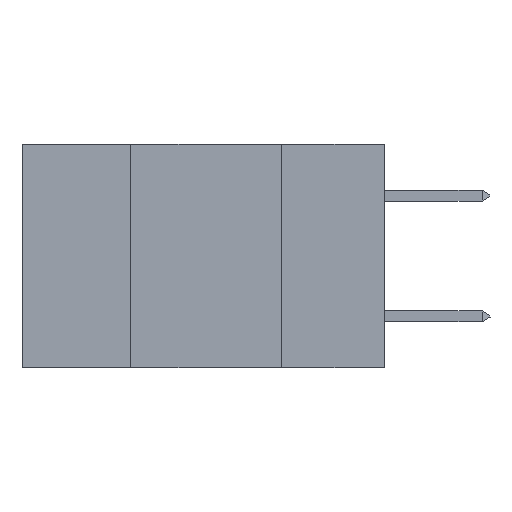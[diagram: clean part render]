
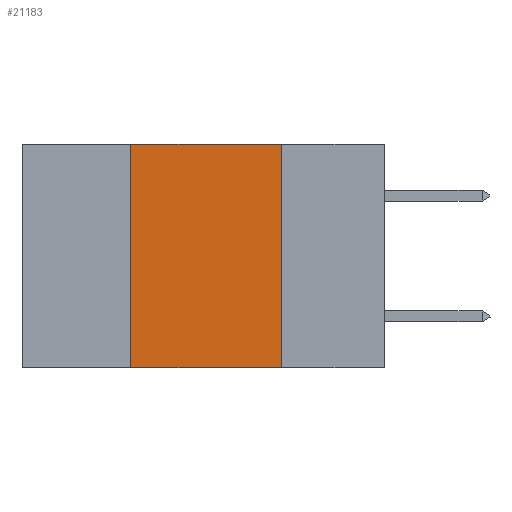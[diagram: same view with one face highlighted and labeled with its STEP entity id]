
A CAD part, left-side view. The second image highlights one B-rep face of the part: STEP entity #21183.
In plain terms, the highlighted planar face has unit normal (-1, 0, 0).
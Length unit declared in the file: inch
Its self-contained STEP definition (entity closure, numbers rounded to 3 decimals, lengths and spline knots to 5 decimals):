
#205 = DIRECTION ( 'NONE',  ( 0., 0., 1. ) ) ;
#1517 = VERTEX_POINT ( 'NONE', #17051 ) ;
#1685 = LINE ( 'NONE', #21232, #7131 ) ;
#1916 = CARTESIAN_POINT ( 'NONE',  ( 0., 0.6, 0. ) ) ;
#2679 = CARTESIAN_POINT ( 'NONE',  ( 0., 0.17, 0. ) ) ;
#4325 = CARTESIAN_POINT ( 'NONE',  ( 0., 0.6, -0.37 ) ) ;
#4379 = ORIENTED_EDGE ( 'NONE', *, *, #7152, .F. ) ;
#6887 = ORIENTED_EDGE ( 'NONE', *, *, #26153, .T. ) ;
#7084 = FACE_OUTER_BOUND ( 'NONE', #20321, .T. ) ;
#7131 = VECTOR ( 'NONE', #15181, 39.37008 ) ;
#7152 = EDGE_CURVE ( 'NONE', #16891, #16046, #12482, .T. ) ;
#7318 = CARTESIAN_POINT ( 'NONE',  ( 0., 0.42, -0.37 ) ) ;
#9005 = LINE ( 'NONE', #14502, #18321 ) ;
#10237 = VERTEX_POINT ( 'NONE', #7318 ) ;
#11109 = EDGE_CURVE ( 'NONE', #16046, #1517, #1685, .T. ) ;
#12009 = EDGE_CURVE ( 'NONE', #10237, #16891, #9005, .T. ) ;
#12128 = DIRECTION ( 'NONE',  ( 1., 0., 0. ) ) ;
#12482 = LINE ( 'NONE', #1916, #14392 ) ;
#13157 = AXIS2_PLACEMENT_3D ( 'NONE', #20233, #12128, #15914 ) ;
#13162 = CARTESIAN_POINT ( 'NONE',  ( 0., 0.42, 0. ) ) ;
#13406 = ORIENTED_EDGE ( 'NONE', *, *, #12009, .F. ) ;
#14392 = VECTOR ( 'NONE', #18538, 39.37008 ) ;
#14502 = CARTESIAN_POINT ( 'NONE',  ( 0., 0.42, 0. ) ) ;
#15181 = DIRECTION ( 'NONE',  ( 0., 0., -1. ) ) ;
#15914 = DIRECTION ( 'NONE',  ( 0., 0., -1. ) ) ;
#16046 = VERTEX_POINT ( 'NONE', #2679 ) ;
#16891 = VERTEX_POINT ( 'NONE', #13162 ) ;
#17051 = CARTESIAN_POINT ( 'NONE',  ( 0., 0.17, -0.37 ) ) ;
#18095 = LINE ( 'NONE', #4325, #22035 ) ;
#18140 = ORIENTED_EDGE ( 'NONE', *, *, #11109, .F. ) ;
#18321 = VECTOR ( 'NONE', #205, 39.37008 ) ;
#18538 = DIRECTION ( 'NONE',  ( 0., -1., 0. ) ) ;
#20233 = CARTESIAN_POINT ( 'NONE',  ( 0., 0.6, 0. ) ) ;
#20321 = EDGE_LOOP ( 'NONE', ( #18140, #4379, #13406, #6887 ) ) ;
#21183 = ADVANCED_FACE ( 'NONE', ( #7084 ), #26581, .F. ) ;
#21232 = CARTESIAN_POINT ( 'NONE',  ( 0., 0.17, 0. ) ) ;
#22035 = VECTOR ( 'NONE', #23069, 39.37008 ) ;
#23069 = DIRECTION ( 'NONE',  ( 0., -1., 0. ) ) ;
#26153 = EDGE_CURVE ( 'NONE', #10237, #1517, #18095, .T. ) ;
#26581 = PLANE ( 'NONE',  #13157 ) ;
